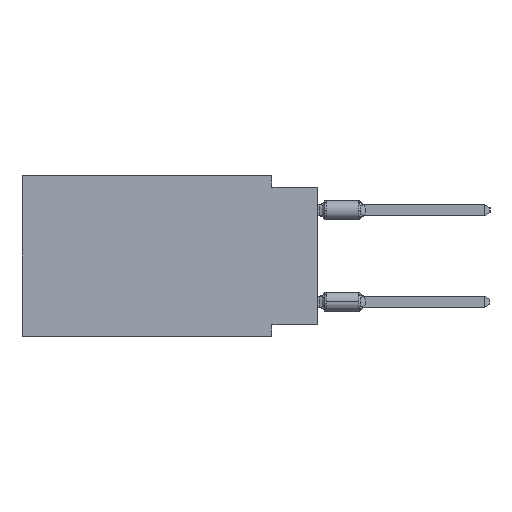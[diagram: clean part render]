
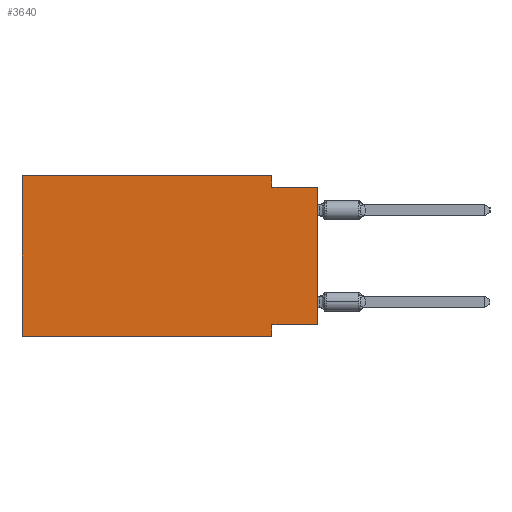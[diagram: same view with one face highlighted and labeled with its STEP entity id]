
A CAD part, left-side view. The second image highlights one B-rep face of the part: STEP entity #3640.
In plain terms, the highlighted planar face has unit normal (-1, 0, 0).
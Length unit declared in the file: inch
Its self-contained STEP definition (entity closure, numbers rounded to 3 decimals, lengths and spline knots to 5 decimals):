
#179 = ORIENTED_EDGE ( 'NONE', *, *, #36269, .F. ) ;
#1266 = EDGE_CURVE ( 'NONE', #41082, #8537, #25666, .T. ) ;
#2066 = CARTESIAN_POINT ( 'NONE',  ( 0., 0.1, 0. ) ) ;
#2124 = CARTESIAN_POINT ( 'NONE',  ( 0., 0., -0.325 ) ) ;
#3216 = DIRECTION ( 'NONE',  ( 0., -1., 0. ) ) ;
#3640 = ADVANCED_FACE ( 'NONE', ( #16105 ), #5079, .F. ) ;
#3708 = EDGE_CURVE ( 'NONE', #41082, #34449, #22972, .T. ) ;
#5079 = PLANE ( 'NONE',  #43543 ) ;
#5536 = CARTESIAN_POINT ( 'NONE',  ( 0., 0.645, 0. ) ) ;
#6621 = LINE ( 'NONE', #20626, #20137 ) ;
#7849 = LINE ( 'NONE', #35756, #38171 ) ;
#8130 = CARTESIAN_POINT ( 'NONE',  ( 0., 0., -0.025 ) ) ;
#8537 = VERTEX_POINT ( 'NONE', #17517 ) ;
#8977 = DIRECTION ( 'NONE',  ( 0., 0., -1. ) ) ;
#9009 = VECTOR ( 'NONE', #39260, 39.37008 ) ;
#9468 = DIRECTION ( 'NONE',  ( 0., 0., -1. ) ) ;
#10140 = CARTESIAN_POINT ( 'NONE',  ( 0., 0.1, -0.35 ) ) ;
#11359 = CARTESIAN_POINT ( 'NONE',  ( 0., 0.1, -0.025 ) ) ;
#11718 = VERTEX_POINT ( 'NONE', #31601 ) ;
#12097 = ORIENTED_EDGE ( 'NONE', *, *, #1266, .T. ) ;
#13746 = EDGE_CURVE ( 'NONE', #27565, #43914, #6621, .T. ) ;
#14288 = CARTESIAN_POINT ( 'NONE',  ( 0., 0.645, -0.35 ) ) ;
#14773 = CARTESIAN_POINT ( 'NONE',  ( 0., 0.1, 0. ) ) ;
#15265 = ORIENTED_EDGE ( 'NONE', *, *, #3708, .F. ) ;
#15541 = VECTOR ( 'NONE', #9468, 39.37008 ) ;
#15667 = VERTEX_POINT ( 'NONE', #14773 ) ;
#15822 = CARTESIAN_POINT ( 'NONE',  ( 0., 0., 0. ) ) ;
#16105 = FACE_OUTER_BOUND ( 'NONE', #22390, .T. ) ;
#17517 = CARTESIAN_POINT ( 'NONE',  ( 0., 0., -0.025 ) ) ;
#19616 = ORIENTED_EDGE ( 'NONE', *, *, #32755, .F. ) ;
#20137 = VECTOR ( 'NONE', #3216, 39.37008 ) ;
#20183 = VECTOR ( 'NONE', #40782, 39.37008 ) ;
#20626 = CARTESIAN_POINT ( 'NONE',  ( 0., 0.645, -0.35 ) ) ;
#21455 = VECTOR ( 'NONE', #25566, 39.37008 ) ;
#21631 = CARTESIAN_POINT ( 'NONE',  ( 0., 0.1, -0.325 ) ) ;
#21826 = DIRECTION ( 'NONE',  ( 0., 0., 1. ) ) ;
#22125 = LINE ( 'NONE', #8130, #21455 ) ;
#22390 = EDGE_LOOP ( 'NONE', ( #12097, #19616, #179, #22478, #39569, #25887, #37371, #15265 ) ) ;
#22478 = ORIENTED_EDGE ( 'NONE', *, *, #32764, .F. ) ;
#22972 = LINE ( 'NONE', #2124, #20183 ) ;
#23217 = CARTESIAN_POINT ( 'NONE',  ( 0., 0., -0.325 ) ) ;
#23623 = VECTOR ( 'NONE', #39585, 39.37008 ) ;
#23824 = VECTOR ( 'NONE', #39196, 39.37008 ) ;
#25566 = DIRECTION ( 'NONE',  ( 0., -1., 0. ) ) ;
#25666 = LINE ( 'NONE', #15822, #23623 ) ;
#25887 = ORIENTED_EDGE ( 'NONE', *, *, #13746, .T. ) ;
#26474 = CARTESIAN_POINT ( 'NONE',  ( 0., 0.1, -0.35 ) ) ;
#27565 = VERTEX_POINT ( 'NONE', #14288 ) ;
#29350 = EDGE_CURVE ( 'NONE', #27565, #11718, #7849, .T. ) ;
#30301 = LINE ( 'NONE', #10140, #15541 ) ;
#31601 = CARTESIAN_POINT ( 'NONE',  ( 0., 0.645, 0. ) ) ;
#32642 = CARTESIAN_POINT ( 'NONE',  ( 0., 0.645, 0. ) ) ;
#32755 = EDGE_CURVE ( 'NONE', #32770, #8537, #22125, .T. ) ;
#32764 = EDGE_CURVE ( 'NONE', #11718, #15667, #33085, .T. ) ;
#32770 = VERTEX_POINT ( 'NONE', #11359 ) ;
#33085 = LINE ( 'NONE', #32642, #9009 ) ;
#34449 = VERTEX_POINT ( 'NONE', #21631 ) ;
#35756 = CARTESIAN_POINT ( 'NONE',  ( 0., 0.645, 0. ) ) ;
#36269 = EDGE_CURVE ( 'NONE', #15667, #32770, #43702, .T. ) ;
#37371 = ORIENTED_EDGE ( 'NONE', *, *, #44533, .F. ) ;
#38171 = VECTOR ( 'NONE', #21826, 39.37008 ) ;
#39196 = DIRECTION ( 'NONE',  ( 0., 0., -1. ) ) ;
#39260 = DIRECTION ( 'NONE',  ( 0., -1., 0. ) ) ;
#39569 = ORIENTED_EDGE ( 'NONE', *, *, #29350, .F. ) ;
#39585 = DIRECTION ( 'NONE',  ( 0., 0., 1. ) ) ;
#40551 = DIRECTION ( 'NONE',  ( 1., 0., 0. ) ) ;
#40782 = DIRECTION ( 'NONE',  ( 0., 1., 0. ) ) ;
#41082 = VERTEX_POINT ( 'NONE', #23217 ) ;
#43543 = AXIS2_PLACEMENT_3D ( 'NONE', #5536, #40551, #8977 ) ;
#43702 = LINE ( 'NONE', #2066, #23824 ) ;
#43914 = VERTEX_POINT ( 'NONE', #26474 ) ;
#44533 = EDGE_CURVE ( 'NONE', #34449, #43914, #30301, .T. ) ;
